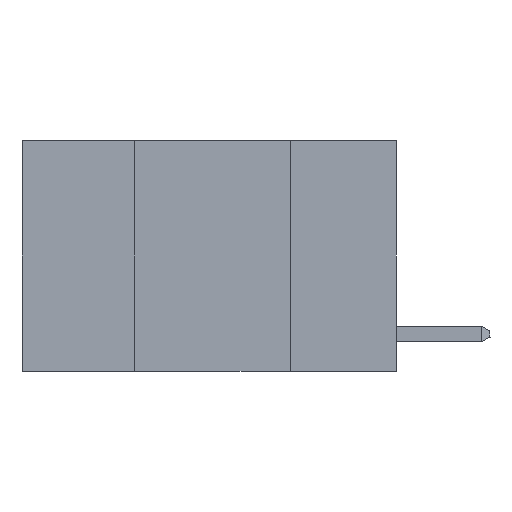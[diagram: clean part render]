
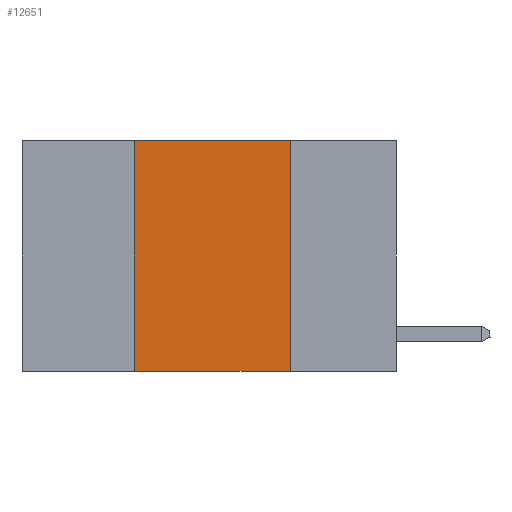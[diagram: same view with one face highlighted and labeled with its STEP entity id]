
A CAD part, left-side view. The second image highlights one B-rep face of the part: STEP entity #12651.
In plain terms, the highlighted planar face has unit normal (-1, 0, 0).
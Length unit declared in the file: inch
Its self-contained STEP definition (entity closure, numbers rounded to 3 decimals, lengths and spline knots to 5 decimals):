
#1745 = DIRECTION ( 'NONE',  ( 0., 0., -1. ) ) ;
#2323 = VECTOR ( 'NONE', #1745, 39.37008 ) ;
#3241 = EDGE_CURVE ( 'NONE', #4685, #24382, #4695, .T. ) ;
#3642 = CARTESIAN_POINT ( 'NONE',  ( 0., 0.42, 0. ) ) ;
#3656 = CARTESIAN_POINT ( 'NONE',  ( 0., 0.17, 0. ) ) ;
#4024 = LINE ( 'NONE', #6029, #14023 ) ;
#4685 = VERTEX_POINT ( 'NONE', #7929 ) ;
#4695 = LINE ( 'NONE', #20165, #22304 ) ;
#6029 = CARTESIAN_POINT ( 'NONE',  ( 0., 0.6, 0. ) ) ;
#6630 = DIRECTION ( 'NONE',  ( 0., 0., -1. ) ) ;
#7432 = LINE ( 'NONE', #3656, #2323 ) ;
#7929 = CARTESIAN_POINT ( 'NONE',  ( 0., 0.42, -0.37 ) ) ;
#8329 = DIRECTION ( 'NONE',  ( 0., 0., 1. ) ) ;
#9178 = CARTESIAN_POINT ( 'NONE',  ( 0., 0.17, 0. ) ) ;
#9862 = CARTESIAN_POINT ( 'NONE',  ( 0., 0.17, -0.37 ) ) ;
#10597 = ORIENTED_EDGE ( 'NONE', *, *, #3241, .T. ) ;
#11413 = CARTESIAN_POINT ( 'NONE',  ( 0., 0.6, 0. ) ) ;
#12102 = ORIENTED_EDGE ( 'NONE', *, *, #17646, .F. ) ;
#12199 = EDGE_LOOP ( 'NONE', ( #14810, #12102, #21355, #10597 ) ) ;
#12651 = ADVANCED_FACE ( 'NONE', ( #24909 ), #22989, .F. ) ;
#13354 = DIRECTION ( 'NONE',  ( 0., -1., 0. ) ) ;
#14023 = VECTOR ( 'NONE', #13354, 39.37008 ) ;
#14036 = CARTESIAN_POINT ( 'NONE',  ( 0., 0.42, 0. ) ) ;
#14679 = EDGE_CURVE ( 'NONE', #16513, #24382, #7432, .T. ) ;
#14810 = ORIENTED_EDGE ( 'NONE', *, *, #14679, .F. ) ;
#16513 = VERTEX_POINT ( 'NONE', #9178 ) ;
#16707 = VERTEX_POINT ( 'NONE', #3642 ) ;
#17646 = EDGE_CURVE ( 'NONE', #16707, #16513, #4024, .T. ) ;
#17745 = LINE ( 'NONE', #14036, #23455 ) ;
#18024 = DIRECTION ( 'NONE',  ( 0., -1., 0. ) ) ;
#18100 = AXIS2_PLACEMENT_3D ( 'NONE', #11413, #19214, #6630 ) ;
#19214 = DIRECTION ( 'NONE',  ( 1., 0., 0. ) ) ;
#20165 = CARTESIAN_POINT ( 'NONE',  ( 0., 0.6, -0.37 ) ) ;
#21355 = ORIENTED_EDGE ( 'NONE', *, *, #22688, .F. ) ;
#22304 = VECTOR ( 'NONE', #18024, 39.37008 ) ;
#22688 = EDGE_CURVE ( 'NONE', #4685, #16707, #17745, .T. ) ;
#22989 = PLANE ( 'NONE',  #18100 ) ;
#23455 = VECTOR ( 'NONE', #8329, 39.37008 ) ;
#24382 = VERTEX_POINT ( 'NONE', #9862 ) ;
#24909 = FACE_OUTER_BOUND ( 'NONE', #12199, .T. ) ;
